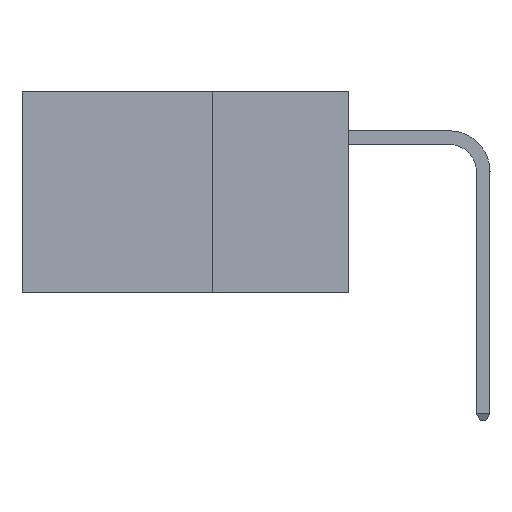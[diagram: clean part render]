
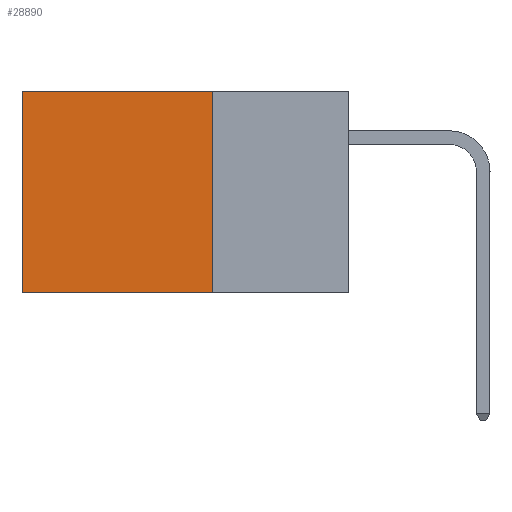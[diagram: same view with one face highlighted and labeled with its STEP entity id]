
A CAD part, left-side view. The second image highlights one B-rep face of the part: STEP entity #28890.
In plain terms, the highlighted planar face has unit normal (-1, 0, 0).
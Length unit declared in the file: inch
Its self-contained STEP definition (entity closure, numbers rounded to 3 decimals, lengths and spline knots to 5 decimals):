
#2736 = DIRECTION ( 'NONE',  ( 0., 0., -1. ) ) ;
#3921 = ORIENTED_EDGE ( 'NONE', *, *, #16693, .F. ) ;
#4535 = VERTEX_POINT ( 'NONE', #17287 ) ;
#4693 = CARTESIAN_POINT ( 'NONE',  ( 0.2875, 0.6, 0. ) ) ;
#5038 = CARTESIAN_POINT ( 'NONE',  ( 0.2875, 0.6, 0. ) ) ;
#7046 = EDGE_CURVE ( 'NONE', #13652, #4535, #30412, .T. ) ;
#12111 = VECTOR ( 'NONE', #16139, 39.37008 ) ;
#13363 = LINE ( 'NONE', #39902, #12111 ) ;
#13652 = VERTEX_POINT ( 'NONE', #4693 ) ;
#14003 = EDGE_CURVE ( 'NONE', #27804, #39372, #31699, .T. ) ;
#15808 = ORIENTED_EDGE ( 'NONE', *, *, #7046, .T. ) ;
#16139 = DIRECTION ( 'NONE',  ( 0., 1., 0. ) ) ;
#16693 = EDGE_CURVE ( 'NONE', #39372, #4535, #13363, .T. ) ;
#17287 = CARTESIAN_POINT ( 'NONE',  ( 0.2875, 0.6, -0.37 ) ) ;
#19576 = DIRECTION ( 'NONE',  ( 1., 0., 0. ) ) ;
#23153 = ORIENTED_EDGE ( 'NONE', *, *, #14003, .F. ) ;
#25801 = CARTESIAN_POINT ( 'NONE',  ( 0.2875, 0.25, 0. ) ) ;
#27425 = CARTESIAN_POINT ( 'NONE',  ( 0.2875, 0.25, 0. ) ) ;
#27804 = VERTEX_POINT ( 'NONE', #25801 ) ;
#28006 = DIRECTION ( 'NONE',  ( 0., 1., 0. ) ) ;
#28890 = ADVANCED_FACE ( 'NONE', ( #38390 ), #43304, .F. ) ;
#30412 = LINE ( 'NONE', #5038, #50100 ) ;
#31699 = LINE ( 'NONE', #50244, #51361 ) ;
#32568 = ORIENTED_EDGE ( 'NONE', *, *, #48709, .T. ) ;
#36696 = DIRECTION ( 'NONE',  ( 0., 0., -1. ) ) ;
#38051 = AXIS2_PLACEMENT_3D ( 'NONE', #27425, #19576, #47267 ) ;
#38390 = FACE_OUTER_BOUND ( 'NONE', #39638, .T. ) ;
#39372 = VERTEX_POINT ( 'NONE', #40799 ) ;
#39638 = EDGE_LOOP ( 'NONE', ( #15808, #3921, #23153, #32568 ) ) ;
#39902 = CARTESIAN_POINT ( 'NONE',  ( 0.2875, 0.25, -0.37 ) ) ;
#40142 = LINE ( 'NONE', #47656, #49341 ) ;
#40799 = CARTESIAN_POINT ( 'NONE',  ( 0.2875, 0.25, -0.37 ) ) ;
#43304 = PLANE ( 'NONE',  #38051 ) ;
#47267 = DIRECTION ( 'NONE',  ( 0., 0., -1. ) ) ;
#47656 = CARTESIAN_POINT ( 'NONE',  ( 0.2875, 0.25, 0. ) ) ;
#48709 = EDGE_CURVE ( 'NONE', #27804, #13652, #40142, .T. ) ;
#49341 = VECTOR ( 'NONE', #28006, 39.37008 ) ;
#50100 = VECTOR ( 'NONE', #36696, 39.37008 ) ;
#50244 = CARTESIAN_POINT ( 'NONE',  ( 0.2875, 0.25, 0. ) ) ;
#51361 = VECTOR ( 'NONE', #2736, 39.37008 ) ;
